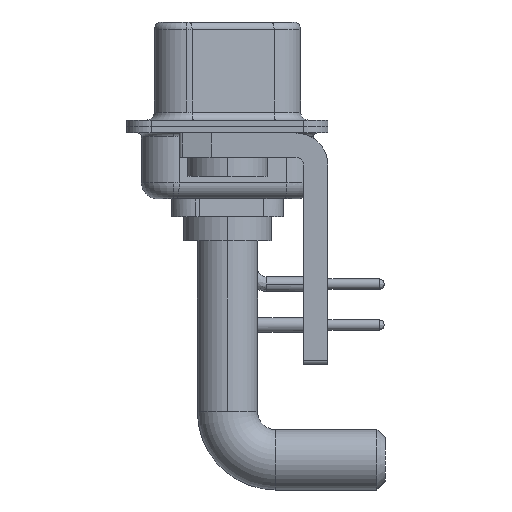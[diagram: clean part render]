
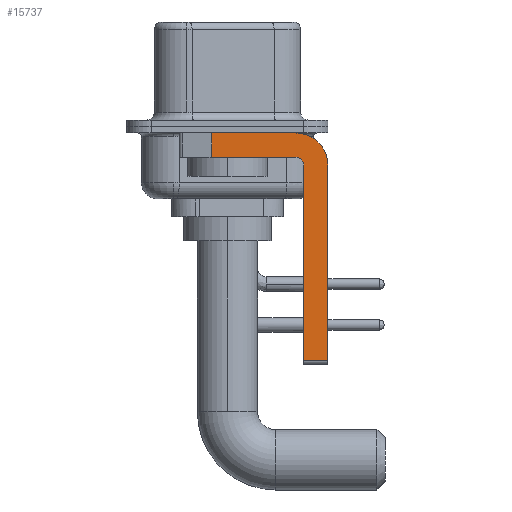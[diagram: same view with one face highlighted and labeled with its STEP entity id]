
A CAD part, left-side view. The second image highlights one B-rep face of the part: STEP entity #15737.
In plain terms, the highlighted planar face has unit normal (-1, 0, 0).
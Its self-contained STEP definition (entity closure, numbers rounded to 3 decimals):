
#284 = VECTOR ( 'NONE', #19594, 1000. ) ;
#285 = DIRECTION ( 'NONE',  ( -1., 0., 0. ) ) ;
#453 = CIRCLE ( 'NONE', #29026, 0.5 ) ;
#1117 = FACE_OUTER_BOUND ( 'NONE', #16663, .T. ) ;
#1443 = VERTEX_POINT ( 'NONE', #24955 ) ;
#2156 = ORIENTED_EDGE ( 'NONE', *, *, #5662, .F. ) ;
#3128 = VECTOR ( 'NONE', #26298, 1000. ) ;
#3416 = DIRECTION ( 'NONE',  ( 0., -1., 0. ) ) ;
#3511 = LINE ( 'NONE', #29008, #284 ) ;
#3678 = EDGE_CURVE ( 'NONE', #17430, #1443, #17197, .T. ) ;
#4184 = ORIENTED_EDGE ( 'NONE', *, *, #16376, .T. ) ;
#4484 = CIRCLE ( 'NONE', #27337, 2. ) ;
#4496 = EDGE_CURVE ( 'NONE', #29439, #13301, #11941, .T. ) ;
#5662 = EDGE_CURVE ( 'NONE', #6600, #10247, #4484, .T. ) ;
#6600 = VERTEX_POINT ( 'NONE', #22841 ) ;
#7085 = ORIENTED_EDGE ( 'NONE', *, *, #3678, .F. ) ;
#7151 = ORIENTED_EDGE ( 'NONE', *, *, #16776, .F. ) ;
#8007 = CARTESIAN_POINT ( 'NONE',  ( -2.9, -6.25, -14.55 ) ) ;
#8909 = EDGE_CURVE ( 'NONE', #10247, #29129, #3511, .T. ) ;
#10229 = DIRECTION ( 'NONE',  ( 0., 0., -1. ) ) ;
#10247 = VERTEX_POINT ( 'NONE', #24575 ) ;
#10539 = CARTESIAN_POINT ( 'NONE',  ( -2.9, -4.75, -14.55 ) ) ;
#11941 = LINE ( 'NONE', #23393, #12367 ) ;
#12367 = VECTOR ( 'NONE', #16972, 1000. ) ;
#12522 = VECTOR ( 'NONE', #3416, 1000. ) ;
#13301 = VERTEX_POINT ( 'NONE', #16130 ) ;
#14477 = ORIENTED_EDGE ( 'NONE', *, *, #8909, .F. ) ;
#14536 = PLANE ( 'NONE',  #26808 ) ;
#15369 = DIRECTION ( 'NONE',  ( 0., 0., -1. ) ) ;
#15737 = ADVANCED_FACE ( 'NONE', ( #1117 ), #14536, .F. ) ;
#15787 = ORIENTED_EDGE ( 'NONE', *, *, #4496, .F. ) ;
#16130 = CARTESIAN_POINT ( 'NONE',  ( -2.9, -4.75, -2.4 ) ) ;
#16376 = EDGE_CURVE ( 'NONE', #29439, #29129, #27557, .T. ) ;
#16403 = LINE ( 'NONE', #21145, #28654 ) ;
#16663 = EDGE_LOOP ( 'NONE', ( #24233, #16754, #7085, #7151, #15787, #4184, #14477, #2156 ) ) ;
#16754 = ORIENTED_EDGE ( 'NONE', *, *, #20115, .T. ) ;
#16776 = EDGE_CURVE ( 'NONE', #13301, #17430, #453, .T. ) ;
#16904 = CARTESIAN_POINT ( 'NONE',  ( -2.9, -4.25, -2.4 ) ) ;
#16972 = DIRECTION ( 'NONE',  ( 0., 0., 1. ) ) ;
#17197 = LINE ( 'NONE', #21367, #3128 ) ;
#17430 = VERTEX_POINT ( 'NONE', #28547 ) ;
#17565 = CARTESIAN_POINT ( 'NONE',  ( -2.9, 3., -0.4 ) ) ;
#18012 = LINE ( 'NONE', #17565, #22848 ) ;
#19018 = DIRECTION ( 'NONE',  ( 0., 0., 1. ) ) ;
#19253 = VERTEX_POINT ( 'NONE', #28114 ) ;
#19594 = DIRECTION ( 'NONE',  ( 0., 0., -1. ) ) ;
#19692 = DIRECTION ( 'NONE',  ( 1., 0., 0. ) ) ;
#19797 = DIRECTION ( 'NONE',  ( 0., -1., 0. ) ) ;
#20115 = EDGE_CURVE ( 'NONE', #19253, #1443, #16403, .T. ) ;
#21145 = CARTESIAN_POINT ( 'NONE',  ( -2.9, 0.978, -1.9 ) ) ;
#21367 = CARTESIAN_POINT ( 'NONE',  ( -2.9, -4.25, -1.9 ) ) ;
#22519 = CARTESIAN_POINT ( 'NONE',  ( -2.9, -4.25, -2.4 ) ) ;
#22841 = CARTESIAN_POINT ( 'NONE',  ( -2.9, -4.25, -0.4 ) ) ;
#22848 = VECTOR ( 'NONE', #19797, 1000. ) ;
#23233 = DIRECTION ( 'NONE',  ( 0., 0., -1. ) ) ;
#23393 = CARTESIAN_POINT ( 'NONE',  ( -2.9, -4.75, -14.8 ) ) ;
#24233 = ORIENTED_EDGE ( 'NONE', *, *, #27641, .F. ) ;
#24575 = CARTESIAN_POINT ( 'NONE',  ( -2.9, -6.25, -2.4 ) ) ;
#24955 = CARTESIAN_POINT ( 'NONE',  ( -2.9, 0.978, -1.9 ) ) ;
#26069 = CARTESIAN_POINT ( 'NONE',  ( -2.9, -4.25, -14.55 ) ) ;
#26298 = DIRECTION ( 'NONE',  ( 0., 1., 0. ) ) ;
#26808 = AXIS2_PLACEMENT_3D ( 'NONE', #16904, #28394, #10229 ) ;
#27337 = AXIS2_PLACEMENT_3D ( 'NONE', #22519, #19692, #15369 ) ;
#27557 = LINE ( 'NONE', #26069, #12522 ) ;
#27641 = EDGE_CURVE ( 'NONE', #19253, #6600, #18012, .T. ) ;
#27852 = CARTESIAN_POINT ( 'NONE',  ( -2.9, -4.25, -2.4 ) ) ;
#28114 = CARTESIAN_POINT ( 'NONE',  ( -2.9, 0.978, -0.4 ) ) ;
#28394 = DIRECTION ( 'NONE',  ( 1., 0., 0. ) ) ;
#28547 = CARTESIAN_POINT ( 'NONE',  ( -2.9, -4.25, -1.9 ) ) ;
#28654 = VECTOR ( 'NONE', #23233, 1000. ) ;
#29008 = CARTESIAN_POINT ( 'NONE',  ( -2.9, -6.25, -2.4 ) ) ;
#29026 = AXIS2_PLACEMENT_3D ( 'NONE', #27852, #285, #19018 ) ;
#29129 = VERTEX_POINT ( 'NONE', #8007 ) ;
#29439 = VERTEX_POINT ( 'NONE', #10539 ) ;
